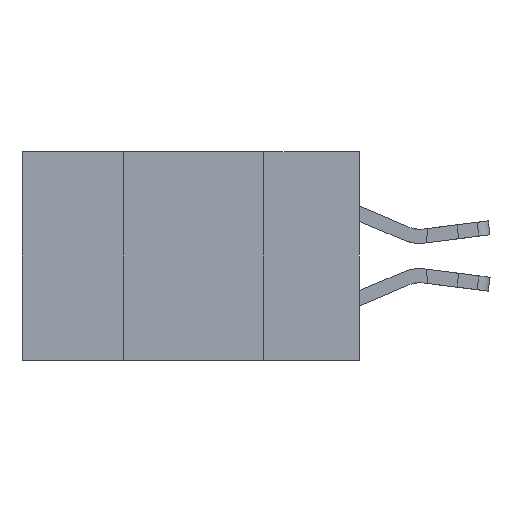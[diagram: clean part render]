
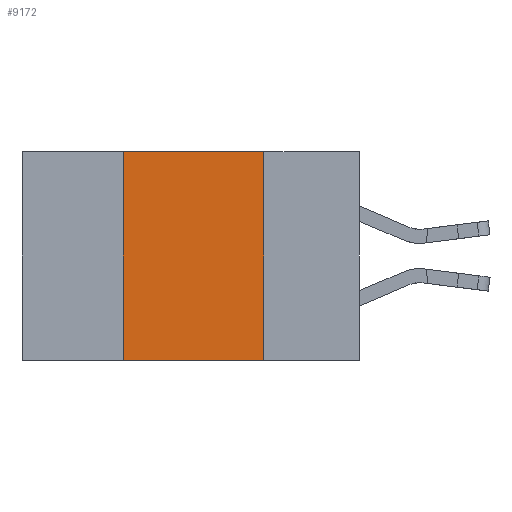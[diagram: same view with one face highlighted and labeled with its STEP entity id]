
A CAD part, left-side view. The second image highlights one B-rep face of the part: STEP entity #9172.
In plain terms, the highlighted planar face has unit normal (-1, 0, 0).
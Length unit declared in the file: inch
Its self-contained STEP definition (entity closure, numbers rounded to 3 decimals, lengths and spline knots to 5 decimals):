
#280 = CARTESIAN_POINT ( 'NONE',  ( 0., 0.6, -0.37 ) ) ;
#1511 = DIRECTION ( 'NONE',  ( 0., 0., -1. ) ) ;
#1611 = EDGE_CURVE ( 'NONE', #20731, #7125, #6361, .T. ) ;
#1687 = CARTESIAN_POINT ( 'NONE',  ( 0., 0.17, 0. ) ) ;
#1808 = ORIENTED_EDGE ( 'NONE', *, *, #19599, .F. ) ;
#2265 = CARTESIAN_POINT ( 'NONE',  ( 0., 0.17, 0. ) ) ;
#3001 = CARTESIAN_POINT ( 'NONE',  ( 0., 0.42, 0. ) ) ;
#3098 = ORIENTED_EDGE ( 'NONE', *, *, #25159, .T. ) ;
#5212 = DIRECTION ( 'NONE',  ( 1., 0., 0. ) ) ;
#6361 = LINE ( 'NONE', #9563, #24904 ) ;
#6594 = ORIENTED_EDGE ( 'NONE', *, *, #1611, .F. ) ;
#6595 = AXIS2_PLACEMENT_3D ( 'NONE', #17889, #5212, #19684 ) ;
#7125 = VERTEX_POINT ( 'NONE', #2265 ) ;
#7802 = VERTEX_POINT ( 'NONE', #24877 ) ;
#8518 = ORIENTED_EDGE ( 'NONE', *, *, #27098, .F. ) ;
#8638 = VECTOR ( 'NONE', #21537, 39.37008 ) ;
#9172 = ADVANCED_FACE ( 'NONE', ( #19077 ), #13610, .F. ) ;
#9563 = CARTESIAN_POINT ( 'NONE',  ( 0., 0.6, 0. ) ) ;
#10928 = LINE ( 'NONE', #280, #8638 ) ;
#11901 = DIRECTION ( 'NONE',  ( 0., 0., 1. ) ) ;
#12854 = VERTEX_POINT ( 'NONE', #13985 ) ;
#13610 = PLANE ( 'NONE',  #6595 ) ;
#13985 = CARTESIAN_POINT ( 'NONE',  ( 0., 0.42, -0.37 ) ) ;
#15018 = VECTOR ( 'NONE', #1511, 39.37008 ) ;
#16259 = EDGE_LOOP ( 'NONE', ( #8518, #6594, #1808, #3098 ) ) ;
#17358 = LINE ( 'NONE', #1687, #15018 ) ;
#17889 = CARTESIAN_POINT ( 'NONE',  ( 0., 0.6, 0. ) ) ;
#19077 = FACE_OUTER_BOUND ( 'NONE', #16259, .T. ) ;
#19389 = VECTOR ( 'NONE', #11901, 39.37008 ) ;
#19599 = EDGE_CURVE ( 'NONE', #12854, #20731, #23069, .T. ) ;
#19684 = DIRECTION ( 'NONE',  ( 0., 0., -1. ) ) ;
#20731 = VERTEX_POINT ( 'NONE', #3001 ) ;
#21537 = DIRECTION ( 'NONE',  ( 0., -1., 0. ) ) ;
#22540 = CARTESIAN_POINT ( 'NONE',  ( 0., 0.42, 0. ) ) ;
#23069 = LINE ( 'NONE', #22540, #19389 ) ;
#24877 = CARTESIAN_POINT ( 'NONE',  ( 0., 0.17, -0.37 ) ) ;
#24904 = VECTOR ( 'NONE', #26667, 39.37008 ) ;
#25159 = EDGE_CURVE ( 'NONE', #12854, #7802, #10928, .T. ) ;
#26667 = DIRECTION ( 'NONE',  ( 0., -1., 0. ) ) ;
#27098 = EDGE_CURVE ( 'NONE', #7125, #7802, #17358, .T. ) ;
